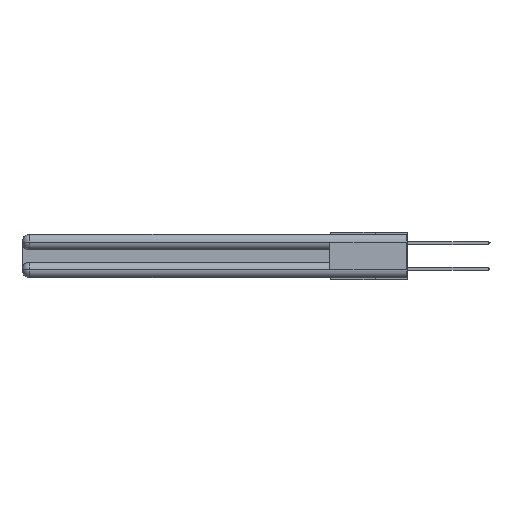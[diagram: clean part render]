
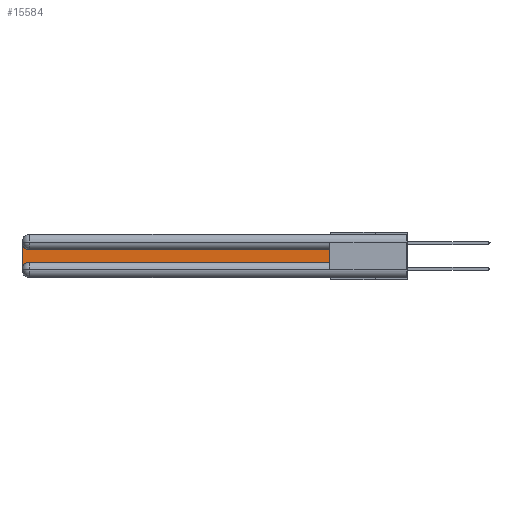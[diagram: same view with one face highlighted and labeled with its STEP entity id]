
A CAD part, left-side view. The second image highlights one B-rep face of the part: STEP entity #15584.
In plain terms, the highlighted planar face has unit normal (-1, 0, 0).
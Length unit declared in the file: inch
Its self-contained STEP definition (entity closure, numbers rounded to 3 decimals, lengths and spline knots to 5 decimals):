
#340 = AXIS2_PLACEMENT_3D ( 'NONE', #27188, #22736, #10662 ) ;
#1086 = ORIENTED_EDGE ( 'NONE', *, *, #30757, .T. ) ;
#2045 = CARTESIAN_POINT ( 'NONE',  ( 0.075, 2.94, -0.0625 ) ) ;
#2558 = CARTESIAN_POINT ( 'NONE',  ( 0.075, 0.6, -0.1225 ) ) ;
#2912 = VERTEX_POINT ( 'NONE', #27636 ) ;
#4685 = VECTOR ( 'NONE', #22406, 39.37008 ) ;
#5151 = CARTESIAN_POINT ( 'NONE',  ( 0.075, 2.94, -0.1225 ) ) ;
#5566 = VERTEX_POINT ( 'NONE', #28940 ) ;
#9573 = DIRECTION ( 'NONE',  ( 0., 0., -1. ) ) ;
#10662 = DIRECTION ( 'NONE',  ( 0., 0., -1. ) ) ;
#11397 = LINE ( 'NONE', #29883, #12930 ) ;
#11754 = VERTEX_POINT ( 'NONE', #13442 ) ;
#11773 = LINE ( 'NONE', #23902, #22759 ) ;
#11836 = ORIENTED_EDGE ( 'NONE', *, *, #18293, .T. ) ;
#12282 = ORIENTED_EDGE ( 'NONE', *, *, #22305, .T. ) ;
#12461 = EDGE_LOOP ( 'NONE', ( #27337, #11836, #26940, #14150, #12282, #1086 ) ) ;
#12855 = VECTOR ( 'NONE', #15470, 39.37008 ) ;
#12930 = VECTOR ( 'NONE', #18060, 39.37008 ) ;
#13442 = CARTESIAN_POINT ( 'NONE',  ( 0.075, 3., -0.2775 ) ) ;
#14150 = ORIENTED_EDGE ( 'NONE', *, *, #24790, .T. ) ;
#14304 = DIRECTION ( 'NONE',  ( 0., 0., 1. ) ) ;
#15133 = EDGE_CURVE ( 'NONE', #23948, #11754, #11397, .T. ) ;
#15470 = DIRECTION ( 'NONE',  ( 0., -1., 0. ) ) ;
#15584 = ADVANCED_FACE ( 'NONE', ( #30311 ), #17885, .F. ) ;
#15746 = LINE ( 'NONE', #2558, #4685 ) ;
#16519 = CARTESIAN_POINT ( 'NONE',  ( 0.075, 3., -0.0625 ) ) ;
#16582 = AXIS2_PLACEMENT_3D ( 'NONE', #26724, #17440, #19774 ) ;
#17440 = DIRECTION ( 'NONE',  ( 1., 0., 0. ) ) ;
#17885 = PLANE ( 'NONE',  #340 ) ;
#18060 = DIRECTION ( 'NONE',  ( 0., 0., -1. ) ) ;
#18293 = EDGE_CURVE ( 'NONE', #22100, #23948, #18421, .T. ) ;
#18421 = CIRCLE ( 'NONE', #25938, 0.06 ) ;
#18459 = EDGE_CURVE ( 'NONE', #5566, #22100, #15746, .T. ) ;
#19774 = DIRECTION ( 'NONE',  ( 0., 0., -1. ) ) ;
#20588 = CIRCLE ( 'NONE', #16582, 0.06 ) ;
#20972 = VERTEX_POINT ( 'NONE', #22855 ) ;
#22100 = VERTEX_POINT ( 'NONE', #5151 ) ;
#22305 = EDGE_CURVE ( 'NONE', #20972, #2912, #27605, .T. ) ;
#22406 = DIRECTION ( 'NONE',  ( 0., 1., 0. ) ) ;
#22736 = DIRECTION ( 'NONE',  ( 1., 0., 0. ) ) ;
#22759 = VECTOR ( 'NONE', #14304, 39.37008 ) ;
#22855 = CARTESIAN_POINT ( 'NONE',  ( 0.075, 2.94, -0.2175 ) ) ;
#23582 = CARTESIAN_POINT ( 'NONE',  ( 0.075, 0.6, -0.2175 ) ) ;
#23902 = CARTESIAN_POINT ( 'NONE',  ( 0.075, 0.6, -0.2175 ) ) ;
#23948 = VERTEX_POINT ( 'NONE', #16519 ) ;
#24081 = DIRECTION ( 'NONE',  ( 1., 0., 0. ) ) ;
#24790 = EDGE_CURVE ( 'NONE', #11754, #20972, #20588, .T. ) ;
#25938 = AXIS2_PLACEMENT_3D ( 'NONE', #2045, #24081, #9573 ) ;
#26724 = CARTESIAN_POINT ( 'NONE',  ( 0.075, 2.94, -0.2775 ) ) ;
#26940 = ORIENTED_EDGE ( 'NONE', *, *, #15133, .T. ) ;
#27188 = CARTESIAN_POINT ( 'NONE',  ( 0.075, 3., -0.1225 ) ) ;
#27337 = ORIENTED_EDGE ( 'NONE', *, *, #18459, .T. ) ;
#27605 = LINE ( 'NONE', #23582, #12855 ) ;
#27636 = CARTESIAN_POINT ( 'NONE',  ( 0.075, 0.6, -0.2175 ) ) ;
#28940 = CARTESIAN_POINT ( 'NONE',  ( 0.075, 0.6, -0.1225 ) ) ;
#29883 = CARTESIAN_POINT ( 'NONE',  ( 0.075, 3., -0.2175 ) ) ;
#30311 = FACE_OUTER_BOUND ( 'NONE', #12461, .T. ) ;
#30757 = EDGE_CURVE ( 'NONE', #2912, #5566, #11773, .T. ) ;
